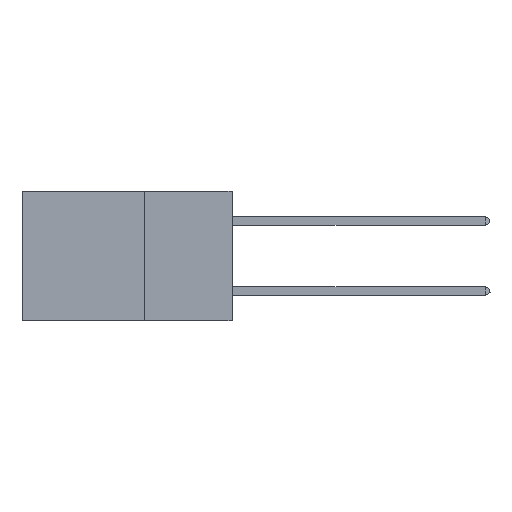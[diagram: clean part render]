
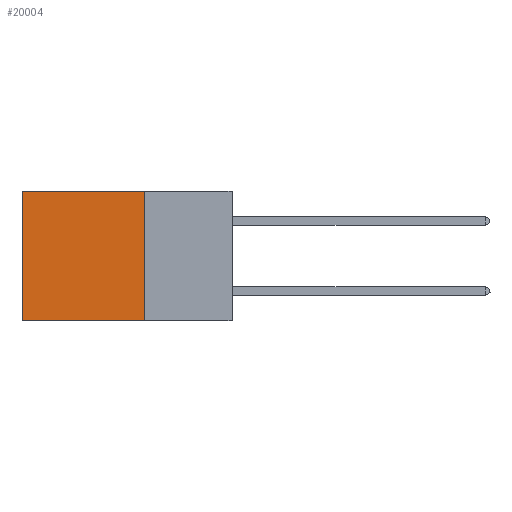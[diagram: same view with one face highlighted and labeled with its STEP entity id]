
A CAD part, left-side view. The second image highlights one B-rep face of the part: STEP entity #20004.
In plain terms, the highlighted planar face has unit normal (-1, 0, 0).
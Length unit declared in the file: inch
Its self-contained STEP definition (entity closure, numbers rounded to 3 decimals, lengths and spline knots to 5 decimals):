
#206 = LINE ( 'NONE', #26613, #9583 ) ;
#438 = ORIENTED_EDGE ( 'NONE', *, *, #29919, .T. ) ;
#1848 = LINE ( 'NONE', #25195, #11976 ) ;
#5023 = ORIENTED_EDGE ( 'NONE', *, *, #20164, .F. ) ;
#8136 = PLANE ( 'NONE',  #32436 ) ;
#8504 = VERTEX_POINT ( 'NONE', #27053 ) ;
#9583 = VECTOR ( 'NONE', #32342, 39.37008 ) ;
#10828 = CARTESIAN_POINT ( 'NONE',  ( 0.2875, 0.25, 0. ) ) ;
#11323 = ORIENTED_EDGE ( 'NONE', *, *, #15054, .F. ) ;
#11976 = VECTOR ( 'NONE', #22312, 39.37008 ) ;
#12347 = DIRECTION ( 'NONE',  ( 0., 0., -1. ) ) ;
#12931 = ORIENTED_EDGE ( 'NONE', *, *, #28837, .T. ) ;
#12997 = DIRECTION ( 'NONE',  ( 1., 0., 0. ) ) ;
#15054 = EDGE_CURVE ( 'NONE', #31025, #33737, #37019, .T. ) ;
#20004 = ADVANCED_FACE ( 'NONE', ( #30215 ), #8136, .F. ) ;
#20164 = EDGE_CURVE ( 'NONE', #33737, #8504, #26710, .T. ) ;
#22312 = DIRECTION ( 'NONE',  ( 0., 0., -1. ) ) ;
#23181 = CARTESIAN_POINT ( 'NONE',  ( 0.2875, 0.25, 0. ) ) ;
#23241 = CARTESIAN_POINT ( 'NONE',  ( 0.2875, 0.25, -0.37 ) ) ;
#25195 = CARTESIAN_POINT ( 'NONE',  ( 0.2875, 0.6, 0. ) ) ;
#26522 = CARTESIAN_POINT ( 'NONE',  ( 0.2875, 0.25, -0.37 ) ) ;
#26613 = CARTESIAN_POINT ( 'NONE',  ( 0.2875, 0.25, 0. ) ) ;
#26710 = LINE ( 'NONE', #26522, #35477 ) ;
#26751 = CARTESIAN_POINT ( 'NONE',  ( 0.2875, 0.6, 0. ) ) ;
#27053 = CARTESIAN_POINT ( 'NONE',  ( 0.2875, 0.6, -0.37 ) ) ;
#27355 = CARTESIAN_POINT ( 'NONE',  ( 0.2875, 0.25, 0. ) ) ;
#28597 = VERTEX_POINT ( 'NONE', #26751 ) ;
#28837 = EDGE_CURVE ( 'NONE', #28597, #8504, #1848, .T. ) ;
#29919 = EDGE_CURVE ( 'NONE', #31025, #28597, #206, .T. ) ;
#30215 = FACE_OUTER_BOUND ( 'NONE', #34618, .T. ) ;
#31025 = VERTEX_POINT ( 'NONE', #23181 ) ;
#32342 = DIRECTION ( 'NONE',  ( 0., 1., 0. ) ) ;
#32436 = AXIS2_PLACEMENT_3D ( 'NONE', #27355, #12997, #37017 ) ;
#32866 = VECTOR ( 'NONE', #12347, 39.37008 ) ;
#33737 = VERTEX_POINT ( 'NONE', #23241 ) ;
#34545 = DIRECTION ( 'NONE',  ( 0., 1., 0. ) ) ;
#34618 = EDGE_LOOP ( 'NONE', ( #12931, #5023, #11323, #438 ) ) ;
#35477 = VECTOR ( 'NONE', #34545, 39.37008 ) ;
#37017 = DIRECTION ( 'NONE',  ( 0., 0., -1. ) ) ;
#37019 = LINE ( 'NONE', #10828, #32866 ) ;
